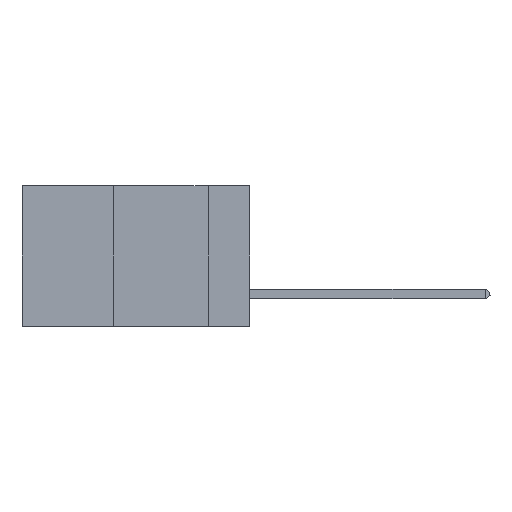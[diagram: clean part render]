
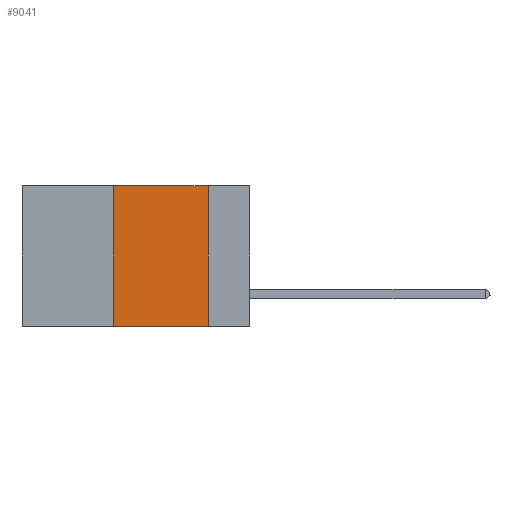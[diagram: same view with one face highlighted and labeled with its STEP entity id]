
A CAD part, left-side view. The second image highlights one B-rep face of the part: STEP entity #9041.
In plain terms, the highlighted planar face has unit normal (-1, 0, 0).
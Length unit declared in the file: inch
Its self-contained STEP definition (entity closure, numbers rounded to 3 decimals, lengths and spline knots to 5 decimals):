
#962 = EDGE_CURVE ( 'NONE', #21622, #13645, #4288, .T. ) ;
#2139 = AXIS2_PLACEMENT_3D ( 'NONE', #8987, #2217, #4065 ) ;
#2217 = DIRECTION ( 'NONE',  ( 1., 0., 0. ) ) ;
#2786 = VECTOR ( 'NONE', #5432, 39.37008 ) ;
#2818 = EDGE_LOOP ( 'NONE', ( #3125, #16062, #10594, #17098 ) ) ;
#2961 = CARTESIAN_POINT ( 'NONE',  ( 0., 0.36, 0. ) ) ;
#3125 = ORIENTED_EDGE ( 'NONE', *, *, #11188, .F. ) ;
#4065 = DIRECTION ( 'NONE',  ( 0., 0., -1. ) ) ;
#4288 = LINE ( 'NONE', #18093, #12700 ) ;
#4770 = CARTESIAN_POINT ( 'NONE',  ( 0., 0.6, -0.37 ) ) ;
#4972 = CARTESIAN_POINT ( 'NONE',  ( 0., 0.11, -0.37 ) ) ;
#5432 = DIRECTION ( 'NONE',  ( 0., -1., 0. ) ) ;
#5440 = LINE ( 'NONE', #4770, #6553 ) ;
#6553 = VECTOR ( 'NONE', #18782, 39.37008 ) ;
#8987 = CARTESIAN_POINT ( 'NONE',  ( 0., 0.6, 0. ) ) ;
#9041 = ADVANCED_FACE ( 'NONE', ( #12985 ), #19302, .F. ) ;
#9345 = CARTESIAN_POINT ( 'NONE',  ( 0., 0.11, 0. ) ) ;
#10126 = LINE ( 'NONE', #10654, #17170 ) ;
#10594 = ORIENTED_EDGE ( 'NONE', *, *, #962, .F. ) ;
#10654 = CARTESIAN_POINT ( 'NONE',  ( 0., 0.11, 0. ) ) ;
#11162 = EDGE_CURVE ( 'NONE', #13645, #17817, #14763, .T. ) ;
#11188 = EDGE_CURVE ( 'NONE', #17817, #11779, #10126, .T. ) ;
#11779 = VERTEX_POINT ( 'NONE', #4972 ) ;
#12256 = DIRECTION ( 'NONE',  ( 0., 0., -1. ) ) ;
#12700 = VECTOR ( 'NONE', #19894, 39.37008 ) ;
#12985 = FACE_OUTER_BOUND ( 'NONE', #2818, .T. ) ;
#13645 = VERTEX_POINT ( 'NONE', #2961 ) ;
#14110 = CARTESIAN_POINT ( 'NONE',  ( 0., 0.6, 0. ) ) ;
#14763 = LINE ( 'NONE', #14110, #2786 ) ;
#16062 = ORIENTED_EDGE ( 'NONE', *, *, #11162, .F. ) ;
#17098 = ORIENTED_EDGE ( 'NONE', *, *, #17156, .T. ) ;
#17119 = CARTESIAN_POINT ( 'NONE',  ( 0., 0.36, -0.37 ) ) ;
#17156 = EDGE_CURVE ( 'NONE', #21622, #11779, #5440, .T. ) ;
#17170 = VECTOR ( 'NONE', #12256, 39.37008 ) ;
#17817 = VERTEX_POINT ( 'NONE', #9345 ) ;
#18093 = CARTESIAN_POINT ( 'NONE',  ( 0., 0.36, 0. ) ) ;
#18782 = DIRECTION ( 'NONE',  ( 0., -1., 0. ) ) ;
#19302 = PLANE ( 'NONE',  #2139 ) ;
#19894 = DIRECTION ( 'NONE',  ( 0., 0., 1. ) ) ;
#21622 = VERTEX_POINT ( 'NONE', #17119 ) ;
